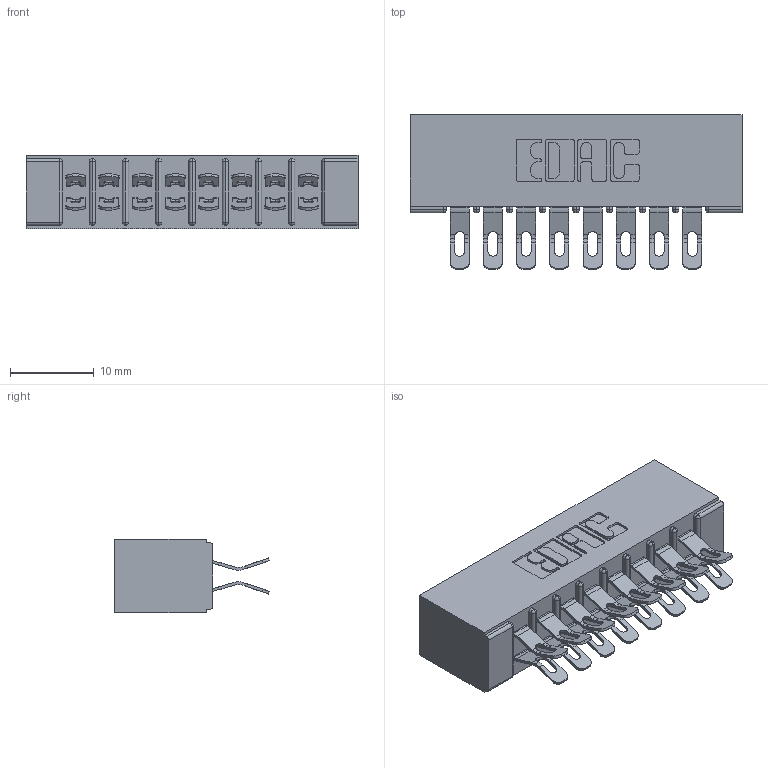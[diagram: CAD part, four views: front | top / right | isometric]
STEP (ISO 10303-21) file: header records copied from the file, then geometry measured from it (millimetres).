
FILE_DESCRIPTION (( 'STEP AP203' ), '1' );
FILE_NAME ('355-016-555-501.STEP', '2019-09-11T02:11:58', ( '' ), ( '' ), 'SwSTEP 2.0', 'SolidWorks 2016', '' );
FILE_SCHEMA (( 'CONFIG_CONTROL_DESIGN' ));
Length unit declared in the file: inch
Products named in the file (3): 305 Part_No Mounting; 305-290-001_555; 355-016-555-501
Assembly tree (17 placements, depth 2):
  355-016-555-501
    305 Part_No Mounting
    305-290-001_555  x16
Bounding box: 39.57 x 18.41 x 8.71 mm (x, y, z)
Volume: 2622.4 mm3; surface area: 5236.6 mm2
Topology: 17 solids, 17 shells, 1164 faces, 3452 edges, 2256 vertices
Faces by surface type: plane 576, cylinder 556, sphere 32
Entity records: 13147 total; most frequent: CARTESIAN_POINT 2192, ORIENTED_EDGE 2160, DIRECTION 2140, EDGE_CURVE 1080, LINE 820, VECTOR 820, VERTEX_POINT 696, AXIS2_PLACEMENT_3D 660
